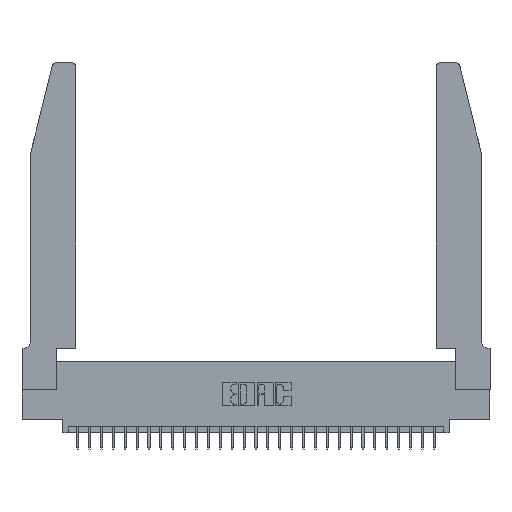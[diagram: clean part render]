
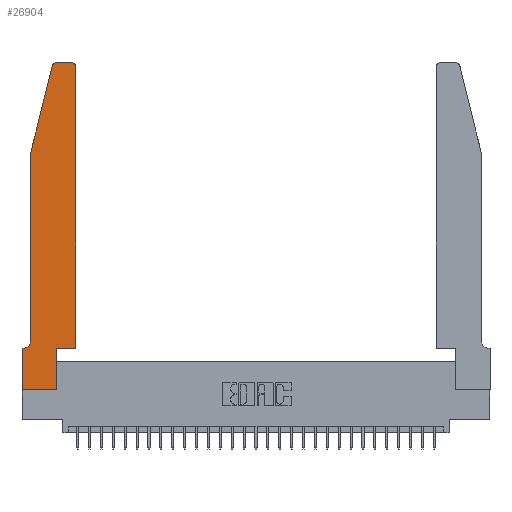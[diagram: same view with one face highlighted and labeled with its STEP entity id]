
A CAD part, top view. The second image highlights one B-rep face of the part: STEP entity #26904.
In plain terms, the highlighted planar face has unit normal (0, 0, 1).
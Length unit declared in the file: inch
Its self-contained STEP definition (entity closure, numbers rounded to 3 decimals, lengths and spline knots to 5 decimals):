
#701 = EDGE_CURVE ( 'NONE', #5640, #28719, #22385, .T. ) ;
#741 = EDGE_CURVE ( 'NONE', #23313, #16685, #19537, .T. ) ;
#970 = ORIENTED_EDGE ( 'NONE', *, *, #741, .T. ) ;
#975 = DIRECTION ( 'NONE',  ( 0., 0., 1. ) ) ;
#1045 = CARTESIAN_POINT ( 'NONE',  ( 0.2605, 2.75, 0.37 ) ) ;
#1200 = LINE ( 'NONE', #27542, #18200 ) ;
#1212 = CARTESIAN_POINT ( 'NONE',  ( 0.25487, 2.72718, 0.37 ) ) ;
#1238 = CARTESIAN_POINT ( 'NONE',  ( 0.284, 2.75, 0.37 ) ) ;
#1290 = CARTESIAN_POINT ( 'NONE',  ( 0.4205, 2.72, 0.37 ) ) ;
#1364 = CARTESIAN_POINT ( 'NONE',  ( 0.4205, 2.75, 0.37 ) ) ;
#1568 = CARTESIAN_POINT ( 'NONE',  ( 0.2865, 0.35, 0.37 ) ) ;
#2529 = LINE ( 'NONE', #7356, #28711 ) ;
#2932 = EDGE_CURVE ( 'NONE', #13567, #8780, #15006, .T. ) ;
#3215 = DIRECTION ( 'NONE',  ( -0.239, -0.971, 0. ) ) ;
#3379 = EDGE_CURVE ( 'NONE', #29046, #23313, #11216, .T. ) ;
#3955 = EDGE_CURVE ( 'NONE', #18171, #29046, #1200, .T. ) ;
#4630 = EDGE_CURVE ( 'NONE', #28719, #25713, #2529, .T. ) ;
#5142 = LINE ( 'NONE', #14643, #28411 ) ;
#5231 = AXIS2_PLACEMENT_3D ( 'NONE', #1290, #975, #8449 ) ;
#5317 = DIRECTION ( 'NONE',  ( 0., -1., 0. ) ) ;
#5449 = DIRECTION ( 'NONE',  ( 1., 0., 0. ) ) ;
#5640 = VERTEX_POINT ( 'NONE', #1212 ) ;
#6016 = CARTESIAN_POINT ( 'NONE',  ( 0.284, 2.72, 0.37 ) ) ;
#6819 = EDGE_CURVE ( 'NONE', #16768, #18171, #5142, .T. ) ;
#7356 = CARTESIAN_POINT ( 'NONE',  ( 0.0755, 2., 0.37 ) ) ;
#7436 = VECTOR ( 'NONE', #24776, 39.37008 ) ;
#7474 = CARTESIAN_POINT ( 'NONE',  ( 0.0755, 0.42, 0.37 ) ) ;
#7782 = FACE_OUTER_BOUND ( 'NONE', #11247, .T. ) ;
#8449 = DIRECTION ( 'NONE',  ( 1., 0., 0. ) ) ;
#8780 = VERTEX_POINT ( 'NONE', #20505 ) ;
#9642 = ORIENTED_EDGE ( 'NONE', *, *, #12524, .T. ) ;
#9963 = LINE ( 'NONE', #19600, #7436 ) ;
#10105 = CARTESIAN_POINT ( 'NONE',  ( 0., 0.35, 0.37 ) ) ;
#10597 = ORIENTED_EDGE ( 'NONE', *, *, #3379, .T. ) ;
#11073 = CARTESIAN_POINT ( 'NONE',  ( 0.0055, 0.42, 0.37 ) ) ;
#11216 = CIRCLE ( 'NONE', #5231, 0.03 ) ;
#11247 = EDGE_LOOP ( 'NONE', ( #970, #18319, #15196, #22735, #9642, #28800, #17890, #12481, #19495, #19534, #17484, #10597 ) ) ;
#11452 = CARTESIAN_POINT ( 'NONE',  ( 0., 0., 0.37 ) ) ;
#11775 = AXIS2_PLACEMENT_3D ( 'NONE', #6016, #29397, #25025 ) ;
#12481 = ORIENTED_EDGE ( 'NONE', *, *, #2932, .T. ) ;
#12524 = EDGE_CURVE ( 'NONE', #25713, #27606, #28554, .T. ) ;
#13567 = VERTEX_POINT ( 'NONE', #11452 ) ;
#13664 = VERTEX_POINT ( 'NONE', #19998 ) ;
#14093 = CARTESIAN_POINT ( 'NONE',  ( 0.0055, 0.35, 0.37 ) ) ;
#14643 = CARTESIAN_POINT ( 'NONE',  ( 0.4505, 0.35, 0.37 ) ) ;
#14892 = CARTESIAN_POINT ( 'NONE',  ( 0.0755, 2., 0.37 ) ) ;
#15006 = LINE ( 'NONE', #20450, #26693 ) ;
#15196 = ORIENTED_EDGE ( 'NONE', *, *, #701, .T. ) ;
#15885 = LINE ( 'NONE', #1568, #24566 ) ;
#16685 = VERTEX_POINT ( 'NONE', #1238 ) ;
#16768 = VERTEX_POINT ( 'NONE', #29429 ) ;
#17100 = DIRECTION ( 'NONE',  ( 0., 0., 1. ) ) ;
#17109 = CARTESIAN_POINT ( 'NONE',  ( 0.0755, 2., 0.37 ) ) ;
#17238 = EDGE_CURVE ( 'NONE', #16685, #5640, #25245, .T. ) ;
#17269 = DIRECTION ( 'NONE',  ( 1., 0., 0. ) ) ;
#17484 = ORIENTED_EDGE ( 'NONE', *, *, #3955, .T. ) ;
#17561 = AXIS2_PLACEMENT_3D ( 'NONE', #11073, #20571, #25571 ) ;
#17589 = DIRECTION ( 'NONE',  ( 0., 1., 0. ) ) ;
#17890 = ORIENTED_EDGE ( 'NONE', *, *, #18486, .T. ) ;
#18171 = VERTEX_POINT ( 'NONE', #23483 ) ;
#18200 = VECTOR ( 'NONE', #25031, 39.37008 ) ;
#18319 = ORIENTED_EDGE ( 'NONE', *, *, #17238, .T. ) ;
#18486 = EDGE_CURVE ( 'NONE', #13664, #13567, #29342, .T. ) ;
#18703 = VECTOR ( 'NONE', #29081, 39.37008 ) ;
#19495 = ORIENTED_EDGE ( 'NONE', *, *, #30370, .T. ) ;
#19534 = ORIENTED_EDGE ( 'NONE', *, *, #6819, .T. ) ;
#19537 = LINE ( 'NONE', #1045, #18703 ) ;
#19600 = CARTESIAN_POINT ( 'NONE',  ( 0.0755, 0.35, 0.37 ) ) ;
#19807 = CARTESIAN_POINT ( 'NONE',  ( 0., 0., 0.37 ) ) ;
#19998 = CARTESIAN_POINT ( 'NONE',  ( 0., 0.35, 0.37 ) ) ;
#20450 = CARTESIAN_POINT ( 'NONE',  ( 0., 0., 0.37 ) ) ;
#20505 = CARTESIAN_POINT ( 'NONE',  ( 0.2865, 0., 0.37 ) ) ;
#20571 = DIRECTION ( 'NONE',  ( 0., 0., -1. ) ) ;
#22385 = LINE ( 'NONE', #14892, #22711 ) ;
#22711 = VECTOR ( 'NONE', #3215, 39.37008 ) ;
#22735 = ORIENTED_EDGE ( 'NONE', *, *, #4630, .T. ) ;
#23313 = VERTEX_POINT ( 'NONE', #1364 ) ;
#23483 = CARTESIAN_POINT ( 'NONE',  ( 0.4505, 0.35, 0.37 ) ) ;
#23767 = CARTESIAN_POINT ( 'NONE',  ( 0.4505, 2.72, 0.37 ) ) ;
#24310 = VECTOR ( 'NONE', #29033, 39.37008 ) ;
#24412 = AXIS2_PLACEMENT_3D ( 'NONE', #10105, #17100, #17269 ) ;
#24566 = VECTOR ( 'NONE', #17589, 39.37008 ) ;
#24776 = DIRECTION ( 'NONE',  ( -1., 0., 0. ) ) ;
#25025 = DIRECTION ( 'NONE',  ( 1., 0., 0. ) ) ;
#25031 = DIRECTION ( 'NONE',  ( 0., 1., 0. ) ) ;
#25245 = CIRCLE ( 'NONE', #11775, 0.03 ) ;
#25571 = DIRECTION ( 'NONE',  ( -1., 0., 0. ) ) ;
#25713 = VERTEX_POINT ( 'NONE', #7474 ) ;
#25854 = EDGE_CURVE ( 'NONE', #27606, #13664, #9963, .T. ) ;
#26693 = VECTOR ( 'NONE', #29974, 39.37008 ) ;
#26904 = ADVANCED_FACE ( 'NONE', ( #7782 ), #29593, .T. ) ;
#27542 = CARTESIAN_POINT ( 'NONE',  ( 0.4505, 0.35, 0.37 ) ) ;
#27606 = VERTEX_POINT ( 'NONE', #14093 ) ;
#28411 = VECTOR ( 'NONE', #5449, 39.37008 ) ;
#28554 = CIRCLE ( 'NONE', #17561, 0.07 ) ;
#28711 = VECTOR ( 'NONE', #5317, 39.37008 ) ;
#28719 = VERTEX_POINT ( 'NONE', #17109 ) ;
#28800 = ORIENTED_EDGE ( 'NONE', *, *, #25854, .T. ) ;
#29033 = DIRECTION ( 'NONE',  ( 0., -1., 0. ) ) ;
#29046 = VERTEX_POINT ( 'NONE', #23767 ) ;
#29081 = DIRECTION ( 'NONE',  ( -1., 0., 0. ) ) ;
#29342 = LINE ( 'NONE', #19807, #24310 ) ;
#29397 = DIRECTION ( 'NONE',  ( 0., 0., 1. ) ) ;
#29429 = CARTESIAN_POINT ( 'NONE',  ( 0.2865, 0.35, 0.37 ) ) ;
#29593 = PLANE ( 'NONE',  #24412 ) ;
#29974 = DIRECTION ( 'NONE',  ( 1., 0., 0. ) ) ;
#30370 = EDGE_CURVE ( 'NONE', #8780, #16768, #15885, .T. ) ;
